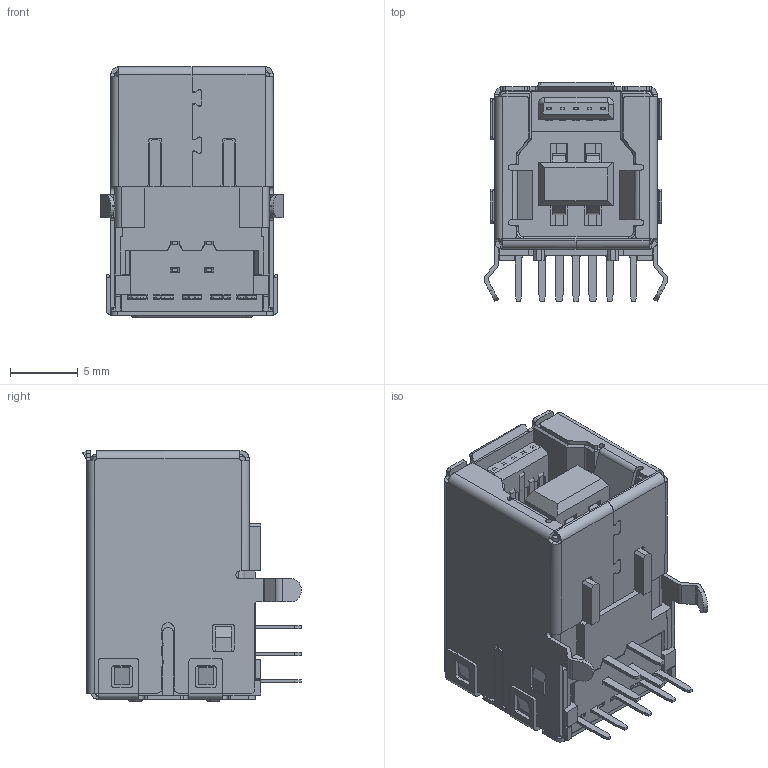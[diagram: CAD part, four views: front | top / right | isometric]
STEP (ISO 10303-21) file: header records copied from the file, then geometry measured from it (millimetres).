
FILE_DESCRIPTION (( 'STEP AP214' ), '1' );
FILE_NAME ('690P209-123-022.STEP', '2021-01-14T20:46:47', ( '' ), ( '' ), 'SwSTEP 2.0', 'SolidWorks 2020', '' );
FILE_SCHEMA (( 'AUTOMOTIVE_DESIGN' ));
Length unit declared in the file: millimetre
Products named in the file (13): Shell 690P209-X23-0XX; Insulator1 690P209-X23-0XX_Blue; Shell2 690P209-X23-0XX; Contact5 690P209-X23-0XX; Insulator3 690P209-X23-0XX_Blue; Contact7 690P209-X23-0XX; Contact2 690P209-X23-0XX; Insulator2 690P209-X23-0XX_Blue; Contact1 690P209-X23-0XX; Contact6 690P209-X23-0XX; Contact9 690P209-X23-0XX; Contact8 690P209-X23-0XX; 690P209-123-022
Assembly tree (14 placements, depth 2):
  690P209-123-022
    Shell 690P209-X23-0XX
    Insulator1 690P209-X23-0XX_Blue
    Contact7 690P209-X23-0XX
    Insulator2 690P209-X23-0XX_Blue
    Contact6 690P209-X23-0XX
    Contact5 690P209-X23-0XX
    Contact8 690P209-X23-0XX
    Contact9 690P209-X23-0XX
    Insulator3 690P209-X23-0XX_Blue
    Shell2 690P209-X23-0XX
    Contact1 690P209-X23-0XX  x2
    Contact2 690P209-X23-0XX  x2
Bounding box: 13.59 x 16.16 x 18.5 mm (x, y, z)
Volume: 1480.9 mm3; surface area: 5358.1 mm2
Topology: 14 solids, 14 shells, 1484 faces, 4150 edges, 2696 vertices
Faces by surface type: plane 1057, cylinder 353, bspline 60, cone 14
Entity records: 46052 total; most frequent: CARTESIAN_POINT 11281, ORIENTED_EDGE 7518, DIRECTION 6507, EDGE_CURVE 3759, VECTOR 2969, LINE 2969, VERTEX_POINT 2438, AXIS2_PLACEMENT_3D 1769
